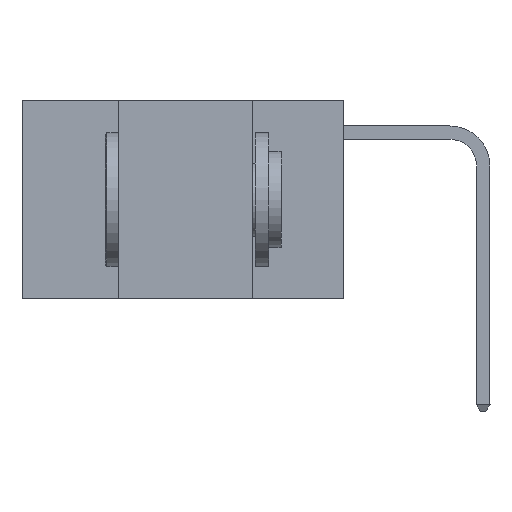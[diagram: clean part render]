
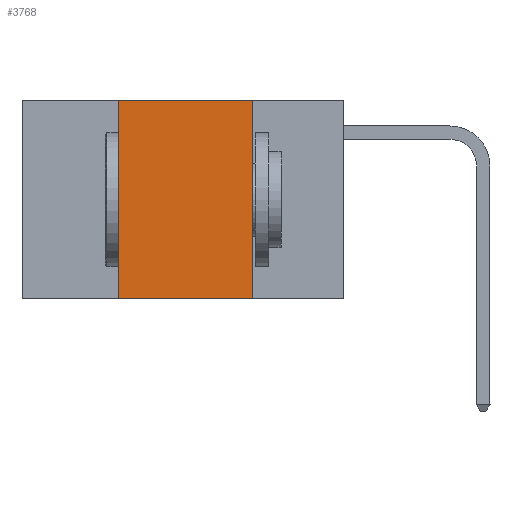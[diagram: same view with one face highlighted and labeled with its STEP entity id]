
A CAD part, left-side view. The second image highlights one B-rep face of the part: STEP entity #3768.
In plain terms, the highlighted planar face has unit normal (-1, 0, 0).
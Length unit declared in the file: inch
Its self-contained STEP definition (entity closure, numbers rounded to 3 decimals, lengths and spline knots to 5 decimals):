
#202 = CARTESIAN_POINT ( 'NONE',  ( 0., 0.42, 0. ) ) ;
#497 = VERTEX_POINT ( 'NONE', #4304 ) ;
#1603 = EDGE_LOOP ( 'NONE', ( #20176, #28017, #19249, #14033 ) ) ;
#2563 = DIRECTION ( 'NONE',  ( 0., 0., 1. ) ) ;
#2771 = PLANE ( 'NONE',  #6525 ) ;
#3768 = ADVANCED_FACE ( 'NONE', ( #21834 ), #2771, .F. ) ;
#4014 = CARTESIAN_POINT ( 'NONE',  ( 0., 0.6, 0. ) ) ;
#4304 = CARTESIAN_POINT ( 'NONE',  ( 0., 0.42, -0.37 ) ) ;
#4585 = VERTEX_POINT ( 'NONE', #15100 ) ;
#4694 = EDGE_CURVE ( 'NONE', #4585, #5160, #21779, .T. ) ;
#5060 = DIRECTION ( 'NONE',  ( 1., 0., 0. ) ) ;
#5160 = VERTEX_POINT ( 'NONE', #5514 ) ;
#5485 = LINE ( 'NONE', #29355, #21711 ) ;
#5514 = CARTESIAN_POINT ( 'NONE',  ( 0., 0.17, 0. ) ) ;
#5959 = EDGE_CURVE ( 'NONE', #497, #29509, #29250, .T. ) ;
#6525 = AXIS2_PLACEMENT_3D ( 'NONE', #28046, #5060, #21193 ) ;
#7475 = LINE ( 'NONE', #202, #25115 ) ;
#8397 = CARTESIAN_POINT ( 'NONE',  ( 0., 0.6, -0.37 ) ) ;
#10862 = VECTOR ( 'NONE', #29138, 39.37008 ) ;
#11559 = EDGE_CURVE ( 'NONE', #5160, #29509, #5485, .T. ) ;
#13338 = CARTESIAN_POINT ( 'NONE',  ( 0., 0.17, -0.37 ) ) ;
#13343 = DIRECTION ( 'NONE',  ( 0., 0., -1. ) ) ;
#14033 = ORIENTED_EDGE ( 'NONE', *, *, #5959, .T. ) ;
#14452 = EDGE_CURVE ( 'NONE', #497, #4585, #7475, .T. ) ;
#15100 = CARTESIAN_POINT ( 'NONE',  ( 0., 0.42, 0. ) ) ;
#15635 = VECTOR ( 'NONE', #20133, 39.37008 ) ;
#19249 = ORIENTED_EDGE ( 'NONE', *, *, #14452, .F. ) ;
#20133 = DIRECTION ( 'NONE',  ( 0., -1., 0. ) ) ;
#20176 = ORIENTED_EDGE ( 'NONE', *, *, #11559, .F. ) ;
#21193 = DIRECTION ( 'NONE',  ( 0., 0., -1. ) ) ;
#21711 = VECTOR ( 'NONE', #13343, 39.37008 ) ;
#21779 = LINE ( 'NONE', #4014, #15635 ) ;
#21834 = FACE_OUTER_BOUND ( 'NONE', #1603, .T. ) ;
#25115 = VECTOR ( 'NONE', #2563, 39.37008 ) ;
#28017 = ORIENTED_EDGE ( 'NONE', *, *, #4694, .F. ) ;
#28046 = CARTESIAN_POINT ( 'NONE',  ( 0., 0.6, 0. ) ) ;
#29138 = DIRECTION ( 'NONE',  ( 0., -1., 0. ) ) ;
#29250 = LINE ( 'NONE', #8397, #10862 ) ;
#29355 = CARTESIAN_POINT ( 'NONE',  ( 0., 0.17, 0. ) ) ;
#29509 = VERTEX_POINT ( 'NONE', #13338 ) ;
